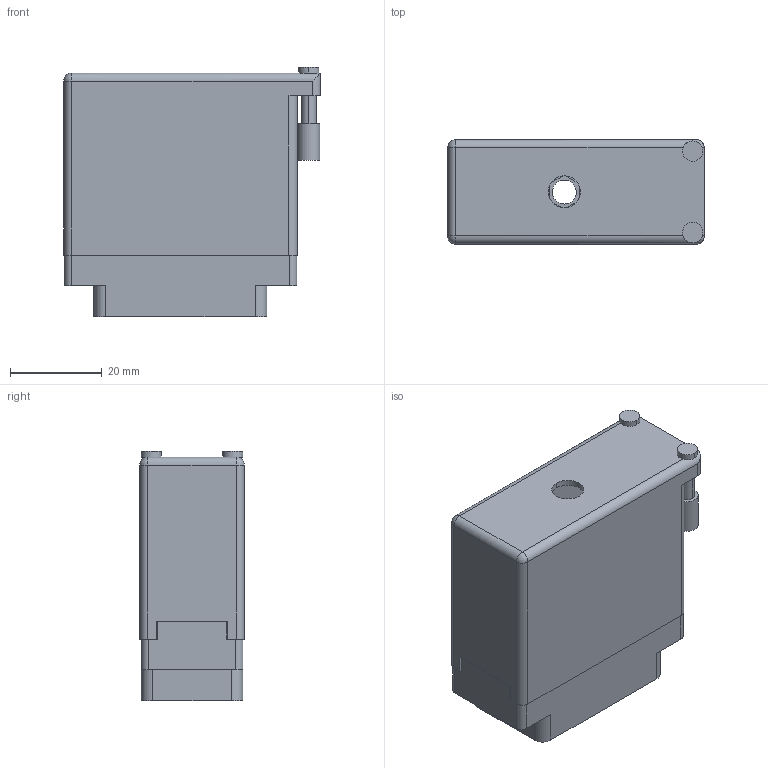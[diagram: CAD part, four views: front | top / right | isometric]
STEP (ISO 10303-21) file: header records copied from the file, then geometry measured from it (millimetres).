
FILE_DESCRIPTION (( 'STEP AP203' ), '1' );
FILE_NAME ('519-036-000-350.STEP', '2020-03-02T21:33:22', ( '' ), ( '' ), 'SwSTEP 2.0', 'SolidWorks 2016', '' );
FILE_SCHEMA (( 'CONFIG_CONTROL_DESIGN' ));
Length unit declared in the file: inch
Products named in the file (3): 516-230-001_Metal - 038 Side Entry; 519-036-000-350; 519 Plug Insulator_036
Assembly tree (2 placements, depth 2):
  519-036-000-350
    519 Plug Insulator_036
    516-230-001_Metal - 038 Side Entry
Bounding box: 56.08 x 22.83 x 54.51 mm (x, y, z)
Volume: 17693.5 mm3; surface area: 24898.1 mm2
Topology: 2 solids, 2 shells, 917 faces, 2674 edges, 1776 vertices
Faces by surface type: plane 648, cylinder 265, cone 2, sphere 2
Entity records: 30833 total; most frequent: CARTESIAN_POINT 5411, ORIENTED_EDGE 5344, DIRECTION 5182, EDGE_CURVE 2672, LINE 1996, VECTOR 1996, VERTEX_POINT 1776, AXIS2_PLACEMENT_3D 1593
